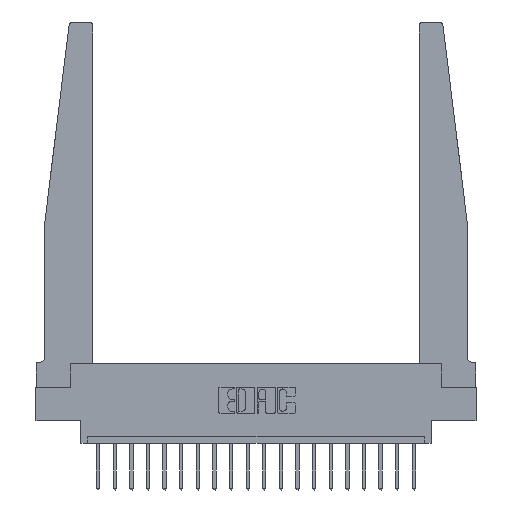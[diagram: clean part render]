
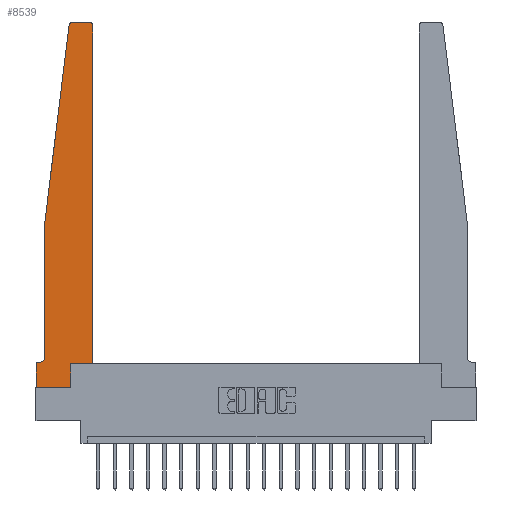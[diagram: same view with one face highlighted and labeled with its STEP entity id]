
A CAD part, top view. The second image highlights one B-rep face of the part: STEP entity #8539.
In plain terms, the highlighted planar face has unit normal (0, 0, 1).
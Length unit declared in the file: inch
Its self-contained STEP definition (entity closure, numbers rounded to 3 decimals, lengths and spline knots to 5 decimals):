
#8 = VERTEX_POINT ( 'NONE', #11743 ) ;
#88 = ORIENTED_EDGE ( 'NONE', *, *, #11261, .T. ) ;
#100 = LINE ( 'NONE', #15859, #14813 ) ;
#422 = VECTOR ( 'NONE', #16015, 39.37008 ) ;
#650 = ORIENTED_EDGE ( 'NONE', *, *, #18959, .T. ) ;
#714 = DIRECTION ( 'NONE',  ( 1., 0., 0. ) ) ;
#1092 = LINE ( 'NONE', #4754, #17264 ) ;
#1253 = DIRECTION ( 'NONE',  ( 0., 0., -1. ) ) ;
#1500 = CARTESIAN_POINT ( 'NONE',  ( 0.395, 2.72, 0.37 ) ) ;
#1826 = CARTESIAN_POINT ( 'NONE',  ( 0.25, 2.75, 0.37 ) ) ;
#2436 = CARTESIAN_POINT ( 'NONE',  ( 0.065, 1.25, 0.37 ) ) ;
#2508 = CARTESIAN_POINT ( 'NONE',  ( 0.065, 1.25, 0.37 ) ) ;
#2819 = CARTESIAN_POINT ( 'NONE',  ( 0.27653, 2.75, 0.37 ) ) ;
#2898 = AXIS2_PLACEMENT_3D ( 'NONE', #12445, #3084, #19926 ) ;
#2915 = EDGE_CURVE ( 'NONE', #17286, #14548, #18749, .T. ) ;
#3039 = CARTESIAN_POINT ( 'NONE',  ( 0.395, 2.75, 0.37 ) ) ;
#3084 = DIRECTION ( 'NONE',  ( 0., 0., 1. ) ) ;
#3242 = ORIENTED_EDGE ( 'NONE', *, *, #2915, .T. ) ;
#3493 = VERTEX_POINT ( 'NONE', #9432 ) ;
#3584 = ORIENTED_EDGE ( 'NONE', *, *, #4031, .T. ) ;
#3675 = VERTEX_POINT ( 'NONE', #3039 ) ;
#4031 = EDGE_CURVE ( 'NONE', #8, #5437, #100, .T. ) ;
#4049 = CARTESIAN_POINT ( 'NONE',  ( 0.425, 2.72, 0.37 ) ) ;
#4064 = CIRCLE ( 'NONE', #12022, 0.03 ) ;
#4325 = CARTESIAN_POINT ( 'NONE',  ( 0.27653, 2.72, 0.37 ) ) ;
#4532 = LINE ( 'NONE', #9844, #422 ) ;
#4754 = CARTESIAN_POINT ( 'NONE',  ( 0.425, 0.18, 0.37 ) ) ;
#4765 = DIRECTION ( 'NONE',  ( 1., 0., 0. ) ) ;
#4893 = CARTESIAN_POINT ( 'NONE',  ( 0., 0., 0.37 ) ) ;
#5269 = DIRECTION ( 'NONE',  ( 0., -1., 0. ) ) ;
#5347 = EDGE_CURVE ( 'NONE', #13765, #8585, #4064, .T. ) ;
#5392 = CARTESIAN_POINT ( 'NONE',  ( 0.015, 0.1875, 0.37 ) ) ;
#5433 = VECTOR ( 'NONE', #10872, 39.37008 ) ;
#5437 = VERTEX_POINT ( 'NONE', #4893 ) ;
#5514 = ORIENTED_EDGE ( 'NONE', *, *, #13234, .T. ) ;
#5826 = DIRECTION ( 'NONE',  ( -1., 0., 0. ) ) ;
#5905 = DIRECTION ( 'NONE',  ( 0., 0., 1. ) ) ;
#6352 = DIRECTION ( 'NONE',  ( -1., 0., 0. ) ) ;
#6424 = EDGE_CURVE ( 'NONE', #6608, #3675, #13592, .T. ) ;
#6608 = VERTEX_POINT ( 'NONE', #4049 ) ;
#7038 = AXIS2_PLACEMENT_3D ( 'NONE', #19840, #1253, #5826 ) ;
#7281 = DIRECTION ( 'NONE',  ( 0., -1., 0. ) ) ;
#7394 = ORIENTED_EDGE ( 'NONE', *, *, #19109, .T. ) ;
#7422 = LINE ( 'NONE', #2436, #9346 ) ;
#7593 = VERTEX_POINT ( 'NONE', #20306 ) ;
#7833 = DIRECTION ( 'NONE',  ( -1., 0., 0. ) ) ;
#7871 = ORIENTED_EDGE ( 'NONE', *, *, #11032, .T. ) ;
#8539 = ADVANCED_FACE ( 'NONE', ( #15979 ), #16848, .T. ) ;
#8585 = VERTEX_POINT ( 'NONE', #14768 ) ;
#9346 = VECTOR ( 'NONE', #15363, 39.37008 ) ;
#9432 = CARTESIAN_POINT ( 'NONE',  ( 0.425, 0.18, 0.37 ) ) ;
#9768 = LINE ( 'NONE', #11399, #10994 ) ;
#9844 = CARTESIAN_POINT ( 'NONE',  ( 0.425, 0.18, 0.37 ) ) ;
#10308 = ORIENTED_EDGE ( 'NONE', *, *, #10483, .T. ) ;
#10483 = EDGE_CURVE ( 'NONE', #11609, #17286, #11413, .T. ) ;
#10643 = VERTEX_POINT ( 'NONE', #15612 ) ;
#10872 = DIRECTION ( 'NONE',  ( 0., 1., 0. ) ) ;
#10994 = VECTOR ( 'NONE', #714, 39.37008 ) ;
#11032 = EDGE_CURVE ( 'NONE', #10643, #3493, #4532, .T. ) ;
#11261 = EDGE_CURVE ( 'NONE', #14548, #8, #20284, .T. ) ;
#11315 = EDGE_CURVE ( 'NONE', #5437, #7593, #9768, .T. ) ;
#11399 = CARTESIAN_POINT ( 'NONE',  ( 0., 0., 0.37 ) ) ;
#11413 = LINE ( 'NONE', #11911, #14134 ) ;
#11609 = VERTEX_POINT ( 'NONE', #2508 ) ;
#11743 = CARTESIAN_POINT ( 'NONE',  ( 0., 0.1875, 0.37 ) ) ;
#11911 = CARTESIAN_POINT ( 'NONE',  ( 0.065, 1.25, 0.37 ) ) ;
#11980 = EDGE_CURVE ( 'NONE', #3675, #13765, #13598, .T. ) ;
#12022 = AXIS2_PLACEMENT_3D ( 'NONE', #4325, #5905, #15339 ) ;
#12075 = ORIENTED_EDGE ( 'NONE', *, *, #5347, .T. ) ;
#12355 = EDGE_LOOP ( 'NONE', ( #14779, #12075, #650, #10308, #3242, #88, #3584, #15983, #5514, #7871, #7394, #13001 ) ) ;
#12445 = CARTESIAN_POINT ( 'NONE',  ( 0., 0.1875, 0.37 ) ) ;
#13001 = ORIENTED_EDGE ( 'NONE', *, *, #6424, .T. ) ;
#13234 = EDGE_CURVE ( 'NONE', #7593, #10643, #16517, .T. ) ;
#13592 = CIRCLE ( 'NONE', #16840, 0.03 ) ;
#13598 = LINE ( 'NONE', #1826, #18494 ) ;
#13765 = VERTEX_POINT ( 'NONE', #2819 ) ;
#14134 = VECTOR ( 'NONE', #7281, 39.37008 ) ;
#14163 = DIRECTION ( 'NONE',  ( 0., 0., 1. ) ) ;
#14548 = VERTEX_POINT ( 'NONE', #5392 ) ;
#14768 = CARTESIAN_POINT ( 'NONE',  ( 0.24675, 2.72367, 0.37 ) ) ;
#14779 = ORIENTED_EDGE ( 'NONE', *, *, #11980, .T. ) ;
#14813 = VECTOR ( 'NONE', #5269, 39.37008 ) ;
#15339 = DIRECTION ( 'NONE',  ( 1., 0., 0. ) ) ;
#15363 = DIRECTION ( 'NONE',  ( -0.122, -0.992, 0. ) ) ;
#15612 = CARTESIAN_POINT ( 'NONE',  ( 0.2605, 0.18, 0.37 ) ) ;
#15859 = CARTESIAN_POINT ( 'NONE',  ( 0., 0., 0.37 ) ) ;
#15979 = FACE_OUTER_BOUND ( 'NONE', #12355, .T. ) ;
#15983 = ORIENTED_EDGE ( 'NONE', *, *, #11315, .T. ) ;
#16015 = DIRECTION ( 'NONE',  ( 1., 0., 0. ) ) ;
#16084 = CARTESIAN_POINT ( 'NONE',  ( 0.065, 0.2375, 0.37 ) ) ;
#16517 = LINE ( 'NONE', #17051, #5433 ) ;
#16840 = AXIS2_PLACEMENT_3D ( 'NONE', #1500, #14163, #4765 ) ;
#16848 = PLANE ( 'NONE',  #2898 ) ;
#17051 = CARTESIAN_POINT ( 'NONE',  ( 0.2605, 0.18, 0.37 ) ) ;
#17264 = VECTOR ( 'NONE', #18743, 39.37008 ) ;
#17286 = VERTEX_POINT ( 'NONE', #16084 ) ;
#17325 = VECTOR ( 'NONE', #6352, 39.37008 ) ;
#18494 = VECTOR ( 'NONE', #7833, 39.37008 ) ;
#18743 = DIRECTION ( 'NONE',  ( 0., 1., 0. ) ) ;
#18749 = CIRCLE ( 'NONE', #7038, 0.05 ) ;
#18959 = EDGE_CURVE ( 'NONE', #8585, #11609, #7422, .T. ) ;
#19109 = EDGE_CURVE ( 'NONE', #3493, #6608, #1092, .T. ) ;
#19128 = CARTESIAN_POINT ( 'NONE',  ( 0.065, 0.1875, 0.37 ) ) ;
#19840 = CARTESIAN_POINT ( 'NONE',  ( 0.015, 0.2375, 0.37 ) ) ;
#19926 = DIRECTION ( 'NONE',  ( 1., 0., 0. ) ) ;
#20284 = LINE ( 'NONE', #19128, #17325 ) ;
#20306 = CARTESIAN_POINT ( 'NONE',  ( 0.2605, 0., 0.37 ) ) ;
